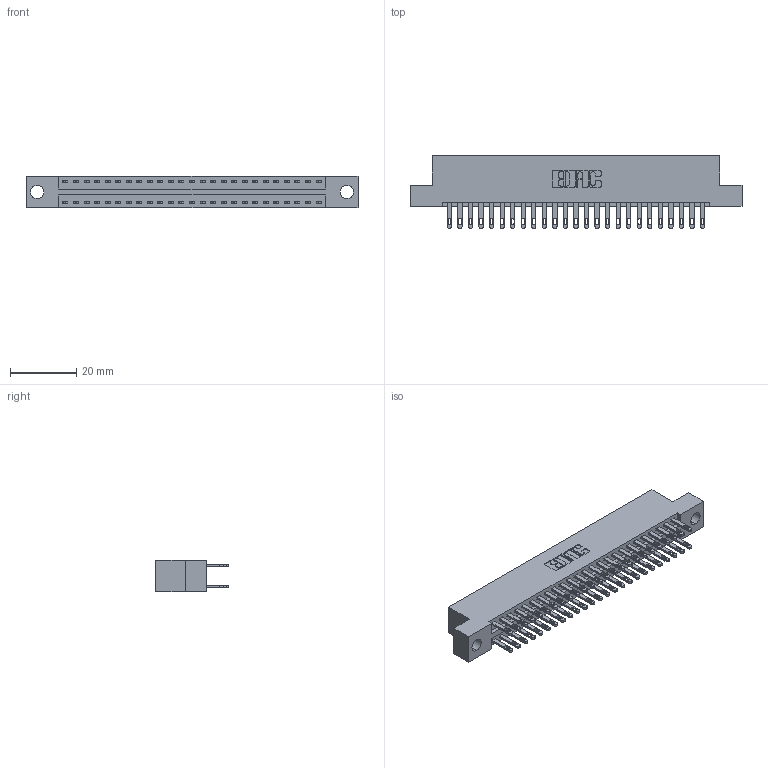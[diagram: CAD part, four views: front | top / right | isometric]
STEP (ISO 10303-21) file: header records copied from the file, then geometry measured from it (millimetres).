
FILE_DESCRIPTION (( 'STEP AP203' ), '1' );
FILE_NAME ('346-050-500-204.STEP', '2022-05-20T22:31:41', ( '' ), ( '' ), 'SwSTEP 2.0', 'SolidWorks 2020', '' );
FILE_SCHEMA (( 'CONFIG_CONTROL_DESIGN' ));
Length unit declared in the file: inch
Products named in the file (3): 346-050-500-204; 346 Part_Flush Mounting Lugs - 0.156 Dia-TH; 345-292-001_345-293-100
Assembly tree (51 placements, depth 2):
  346-050-500-204
    346 Part_Flush Mounting Lugs - 0.156 Dia-TH
    345-292-001_345-293-100  x50
Bounding box: 99.95 x 21.84 x 9.4 mm (x, y, z)
Volume: 9661.1 mm3; surface area: 13383.8 mm2
Topology: 51 solids, 51 shells, 2536 faces, 7715 edges, 5142 vertices
Faces by surface type: plane 1540, cylinder 996
Entity records: 18953 total; most frequent: CARTESIAN_POINT 3150, ORIENTED_EDGE 3082, DIRECTION 2829, EDGE_CURVE 1541, VECTOR 1305, LINE 1305, VERTEX_POINT 1026, AXIS2_PLACEMENT_3D 762
